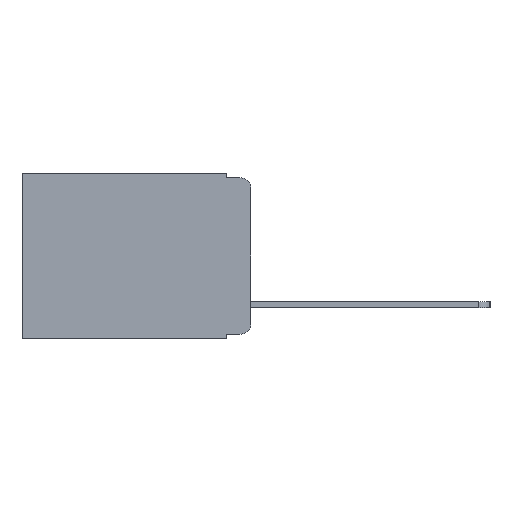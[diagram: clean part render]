
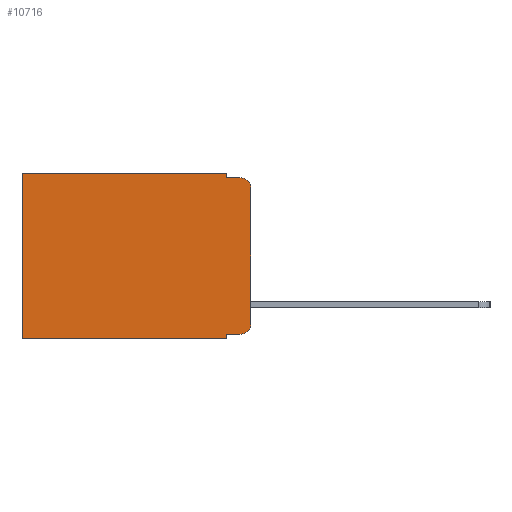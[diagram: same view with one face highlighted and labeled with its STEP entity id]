
A CAD part, left-side view. The second image highlights one B-rep face of the part: STEP entity #10716.
In plain terms, the highlighted planar face has unit normal (-1, 0, 0).
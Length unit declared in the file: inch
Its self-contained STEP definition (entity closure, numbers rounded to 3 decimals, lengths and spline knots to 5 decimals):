
#113 = CARTESIAN_POINT ( 'NONE',  ( 0.298, 0., 0. ) ) ;
#159 = CARTESIAN_POINT ( 'NONE',  ( 0.298, 0.051, -0.343 ) ) ;
#454 = ORIENTED_EDGE ( 'NONE', *, *, #5413, .T. ) ;
#468 = VECTOR ( 'NONE', #10233, 39.37008 ) ;
#474 = PLANE ( 'NONE',  #1285 ) ;
#716 = CARTESIAN_POINT ( 'NONE',  ( 0.298, 0.02, -0.333 ) ) ;
#766 = LINE ( 'NONE', #113, #468 ) ;
#804 = LINE ( 'NONE', #3807, #6455 ) ;
#874 = ORIENTED_EDGE ( 'NONE', *, *, #3190, .F. ) ;
#1000 = CIRCLE ( 'NONE', #8630, 0.02 ) ;
#1285 = AXIS2_PLACEMENT_3D ( 'NONE', #6166, #3380, #9784 ) ;
#1291 = EDGE_CURVE ( 'NONE', #7780, #11418, #5016, .T. ) ;
#1310 = CARTESIAN_POINT ( 'NONE',  ( 0.298, 0.051, -0.01 ) ) ;
#1323 = VERTEX_POINT ( 'NONE', #716 ) ;
#1325 = AXIS2_PLACEMENT_3D ( 'NONE', #7630, #2057, #8549 ) ;
#1367 = CARTESIAN_POINT ( 'NONE',  ( 0.298, 0., 0. ) ) ;
#1379 = CARTESIAN_POINT ( 'NONE',  ( 0.298, 0.051, -0.333 ) ) ;
#2057 = DIRECTION ( 'NONE',  ( -1., 0., 0. ) ) ;
#2398 = ORIENTED_EDGE ( 'NONE', *, *, #5255, .F. ) ;
#2479 = VECTOR ( 'NONE', #11627, 39.37008 ) ;
#2585 = CARTESIAN_POINT ( 'NONE',  ( 0.298, 0.473, 0. ) ) ;
#2668 = CARTESIAN_POINT ( 'NONE',  ( 0.298, 0., -0.343 ) ) ;
#3080 = VERTEX_POINT ( 'NONE', #10929 ) ;
#3178 = DIRECTION ( 'NONE',  ( 0., 0., -1. ) ) ;
#3190 = EDGE_CURVE ( 'NONE', #3080, #6624, #766, .T. ) ;
#3380 = DIRECTION ( 'NONE',  ( 1., 0., 0. ) ) ;
#3387 = DIRECTION ( 'NONE',  ( 0., 0., -1. ) ) ;
#3649 = DIRECTION ( 'NONE',  ( 0., 1., 0. ) ) ;
#3807 = CARTESIAN_POINT ( 'NONE',  ( 0.298, 0.051, 0. ) ) ;
#4227 = VECTOR ( 'NONE', #7840, 39.37008 ) ;
#4345 = EDGE_CURVE ( 'NONE', #11418, #6864, #7491, .T. ) ;
#4394 = ORIENTED_EDGE ( 'NONE', *, *, #6647, .F. ) ;
#4646 = CARTESIAN_POINT ( 'NONE',  ( 0.298, 0.02, -0.03 ) ) ;
#4793 = VECTOR ( 'NONE', #3387, 39.37008 ) ;
#5016 = LINE ( 'NONE', #1367, #2479 ) ;
#5080 = CARTESIAN_POINT ( 'NONE',  ( 0.298, 0.051, 0. ) ) ;
#5255 = EDGE_CURVE ( 'NONE', #8945, #8774, #804, .T. ) ;
#5407 = LINE ( 'NONE', #2668, #7806 ) ;
#5413 = EDGE_CURVE ( 'NONE', #1323, #6624, #8992, .T. ) ;
#5553 = DIRECTION ( 'NONE',  ( 0., 0., -1. ) ) ;
#5698 = CARTESIAN_POINT ( 'NONE',  ( 0.298, 0.02, -0.01 ) ) ;
#5719 = CARTESIAN_POINT ( 'NONE',  ( 0.298, 0.473, -0.343 ) ) ;
#5731 = VERTEX_POINT ( 'NONE', #11585 ) ;
#6083 = CARTESIAN_POINT ( 'NONE',  ( 0.298, 0.051, -0.333 ) ) ;
#6166 = CARTESIAN_POINT ( 'NONE',  ( 0.298, 0., 0. ) ) ;
#6379 = ORIENTED_EDGE ( 'NONE', *, *, #1291, .T. ) ;
#6438 = EDGE_LOOP ( 'NONE', ( #874, #10741, #8919, #7365, #6379, #6524, #4394, #2398, #9766, #454 ) ) ;
#6455 = VECTOR ( 'NONE', #11065, 39.37008 ) ;
#6524 = ORIENTED_EDGE ( 'NONE', *, *, #4345, .T. ) ;
#6624 = VERTEX_POINT ( 'NONE', #9970 ) ;
#6647 = EDGE_CURVE ( 'NONE', #8774, #6864, #5407, .T. ) ;
#6785 = CARTESIAN_POINT ( 'NONE',  ( 0.298, 0.051, 0. ) ) ;
#6813 = CARTESIAN_POINT ( 'NONE',  ( 0.298, 0.473, 0. ) ) ;
#6864 = VERTEX_POINT ( 'NONE', #5719 ) ;
#6942 = VECTOR ( 'NONE', #3178, 39.37008 ) ;
#7230 = EDGE_CURVE ( 'NONE', #8945, #1323, #7797, .T. ) ;
#7365 = ORIENTED_EDGE ( 'NONE', *, *, #9437, .F. ) ;
#7491 = LINE ( 'NONE', #2585, #4793 ) ;
#7630 = CARTESIAN_POINT ( 'NONE',  ( 0.298, 0.02, -0.313 ) ) ;
#7648 = VERTEX_POINT ( 'NONE', #5698 ) ;
#7780 = VERTEX_POINT ( 'NONE', #6785 ) ;
#7797 = LINE ( 'NONE', #6083, #9917 ) ;
#7806 = VECTOR ( 'NONE', #3649, 39.37008 ) ;
#7840 = DIRECTION ( 'NONE',  ( 0., -1., 0. ) ) ;
#8549 = DIRECTION ( 'NONE',  ( 0., 0., -1. ) ) ;
#8630 = AXIS2_PLACEMENT_3D ( 'NONE', #4646, #10971, #5553 ) ;
#8774 = VERTEX_POINT ( 'NONE', #159 ) ;
#8919 = ORIENTED_EDGE ( 'NONE', *, *, #9475, .F. ) ;
#8945 = VERTEX_POINT ( 'NONE', #1379 ) ;
#8992 = CIRCLE ( 'NONE', #1325, 0.02 ) ;
#9303 = FACE_OUTER_BOUND ( 'NONE', #6438, .T. ) ;
#9335 = LINE ( 'NONE', #1310, #4227 ) ;
#9437 = EDGE_CURVE ( 'NONE', #7780, #5731, #9609, .T. ) ;
#9475 = EDGE_CURVE ( 'NONE', #5731, #7648, #9335, .T. ) ;
#9609 = LINE ( 'NONE', #5080, #6942 ) ;
#9766 = ORIENTED_EDGE ( 'NONE', *, *, #7230, .T. ) ;
#9784 = DIRECTION ( 'NONE',  ( 0., 0., -1. ) ) ;
#9917 = VECTOR ( 'NONE', #11487, 39.37008 ) ;
#9970 = CARTESIAN_POINT ( 'NONE',  ( 0.298, 0., -0.313 ) ) ;
#10233 = DIRECTION ( 'NONE',  ( 0., 0., -1. ) ) ;
#10408 = EDGE_CURVE ( 'NONE', #3080, #7648, #1000, .T. ) ;
#10716 = ADVANCED_FACE ( 'NONE', ( #9303 ), #474, .F. ) ;
#10741 = ORIENTED_EDGE ( 'NONE', *, *, #10408, .T. ) ;
#10929 = CARTESIAN_POINT ( 'NONE',  ( 0.298, 0., -0.03 ) ) ;
#10971 = DIRECTION ( 'NONE',  ( -1., 0., 0. ) ) ;
#11065 = DIRECTION ( 'NONE',  ( 0., 0., -1. ) ) ;
#11418 = VERTEX_POINT ( 'NONE', #6813 ) ;
#11487 = DIRECTION ( 'NONE',  ( 0., -1., 0. ) ) ;
#11585 = CARTESIAN_POINT ( 'NONE',  ( 0.298, 0.051, -0.01 ) ) ;
#11627 = DIRECTION ( 'NONE',  ( 0., 1., 0. ) ) ;
